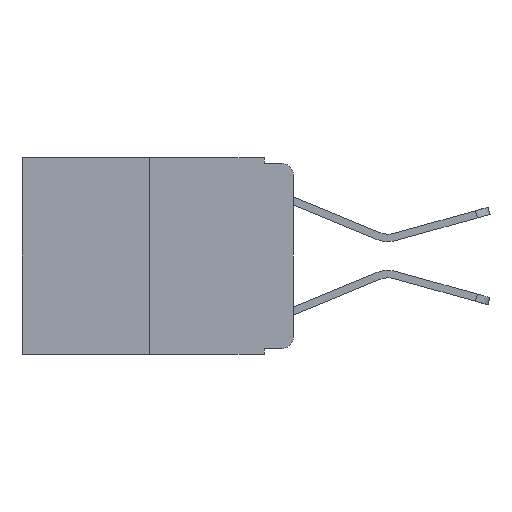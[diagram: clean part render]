
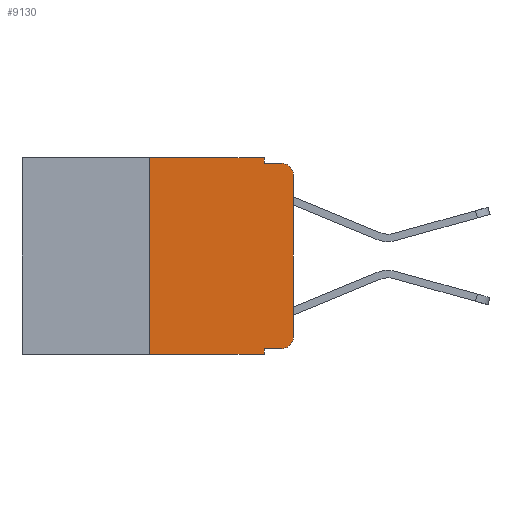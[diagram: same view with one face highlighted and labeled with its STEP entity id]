
A CAD part, left-side view. The second image highlights one B-rep face of the part: STEP entity #9130.
In plain terms, the highlighted planar face has unit normal (-1, 0, 0).
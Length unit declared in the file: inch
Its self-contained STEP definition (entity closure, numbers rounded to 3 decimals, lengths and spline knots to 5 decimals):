
#79 = EDGE_CURVE ( 'NONE', #3912, #1790, #16710, .T. ) ;
#196 = EDGE_CURVE ( 'NONE', #3220, #19184, #2141, .T. ) ;
#398 = CIRCLE ( 'NONE', #16235, 0.02 ) ;
#466 = CARTESIAN_POINT ( 'NONE',  ( 0., 0.051, -0.343 ) ) ;
#567 = LINE ( 'NONE', #5723, #11896 ) ;
#757 = CARTESIAN_POINT ( 'NONE',  ( 0., 0.02, -0.01 ) ) ;
#910 = VECTOR ( 'NONE', #4980, 39.37008 ) ;
#1705 = EDGE_CURVE ( 'NONE', #19184, #5150, #398, .T. ) ;
#1753 = CARTESIAN_POINT ( 'NONE',  ( 0., 0.02, -0.313 ) ) ;
#1790 = VERTEX_POINT ( 'NONE', #10954 ) ;
#2141 = LINE ( 'NONE', #2347, #18824 ) ;
#2221 = CIRCLE ( 'NONE', #15056, 0.02 ) ;
#2347 = CARTESIAN_POINT ( 'NONE',  ( 0., 0., 0. ) ) ;
#2667 = VERTEX_POINT ( 'NONE', #8052 ) ;
#2764 = VERTEX_POINT ( 'NONE', #10060 ) ;
#2917 = EDGE_CURVE ( 'NONE', #1790, #2667, #15469, .T. ) ;
#3115 = EDGE_CURVE ( 'NONE', #19830, #5150, #12165, .T. ) ;
#3220 = VERTEX_POINT ( 'NONE', #14313 ) ;
#3328 = DIRECTION ( 'NONE',  ( 0., 0., -1. ) ) ;
#3658 = CARTESIAN_POINT ( 'NONE',  ( 0., 0.051, -0.01 ) ) ;
#3828 = LINE ( 'NONE', #4801, #15465 ) ;
#3912 = VERTEX_POINT ( 'NONE', #14672 ) ;
#3943 = EDGE_LOOP ( 'NONE', ( #16195, #19051, #5793, #12200, #5073, #11214, #19737, #18551, #5307, #17861 ) ) ;
#4109 = VECTOR ( 'NONE', #18188, 39.37008 ) ;
#4532 = DIRECTION ( 'NONE',  ( 0., 0., -1. ) ) ;
#4801 = CARTESIAN_POINT ( 'NONE',  ( 0., 0.473, -0.343 ) ) ;
#4980 = DIRECTION ( 'NONE',  ( 0., -1., 0. ) ) ;
#5073 = ORIENTED_EDGE ( 'NONE', *, *, #2917, .F. ) ;
#5096 = LINE ( 'NONE', #11083, #910 ) ;
#5150 = VERTEX_POINT ( 'NONE', #757 ) ;
#5304 = DIRECTION ( 'NONE',  ( -1., 0., 0. ) ) ;
#5307 = ORIENTED_EDGE ( 'NONE', *, *, #13501, .T. ) ;
#5723 = CARTESIAN_POINT ( 'NONE',  ( 0., 0.051, 0. ) ) ;
#5793 = ORIENTED_EDGE ( 'NONE', *, *, #3115, .F. ) ;
#5975 = FACE_OUTER_BOUND ( 'NONE', #3943, .T. ) ;
#7239 = DIRECTION ( 'NONE',  ( 0., 0., -1. ) ) ;
#7643 = CARTESIAN_POINT ( 'NONE',  ( 0., 0., -0.03 ) ) ;
#7645 = VECTOR ( 'NONE', #17916, 39.37008 ) ;
#8049 = CARTESIAN_POINT ( 'NONE',  ( 0., 0.02, -0.03 ) ) ;
#8052 = CARTESIAN_POINT ( 'NONE',  ( 0., 0.051, 0. ) ) ;
#9011 = CARTESIAN_POINT ( 'NONE',  ( 0., 0.473, 0. ) ) ;
#9125 = CARTESIAN_POINT ( 'NONE',  ( 0., 0.473, 0. ) ) ;
#9130 = ADVANCED_FACE ( 'NONE', ( #5975 ), #10528, .F. ) ;
#9292 = EDGE_CURVE ( 'NONE', #2764, #12042, #19494, .T. ) ;
#9357 = DIRECTION ( 'NONE',  ( 0., 0., 1. ) ) ;
#10060 = CARTESIAN_POINT ( 'NONE',  ( 0., 0.051, -0.333 ) ) ;
#10528 = PLANE ( 'NONE',  #18271 ) ;
#10664 = DIRECTION ( 'NONE',  ( 0., 0., -1. ) ) ;
#10954 = CARTESIAN_POINT ( 'NONE',  ( 0., 0.25, 0. ) ) ;
#11083 = CARTESIAN_POINT ( 'NONE',  ( 0., 0.051, -0.333 ) ) ;
#11214 = ORIENTED_EDGE ( 'NONE', *, *, #79, .F. ) ;
#11450 = VECTOR ( 'NONE', #15600, 39.37008 ) ;
#11454 = VECTOR ( 'NONE', #15823, 39.37008 ) ;
#11896 = VECTOR ( 'NONE', #7239, 39.37008 ) ;
#12042 = VERTEX_POINT ( 'NONE', #466 ) ;
#12165 = LINE ( 'NONE', #18536, #7645 ) ;
#12200 = ORIENTED_EDGE ( 'NONE', *, *, #19418, .F. ) ;
#12483 = DIRECTION ( 'NONE',  ( -1., 0., 0. ) ) ;
#13286 = VERTEX_POINT ( 'NONE', #15776 ) ;
#13501 = EDGE_CURVE ( 'NONE', #2764, #13286, #5096, .T. ) ;
#13894 = DIRECTION ( 'NONE',  ( 0., -1., 0. ) ) ;
#14089 = CARTESIAN_POINT ( 'NONE',  ( 0., 0.051, 0. ) ) ;
#14313 = CARTESIAN_POINT ( 'NONE',  ( 0., 0., -0.313 ) ) ;
#14672 = CARTESIAN_POINT ( 'NONE',  ( 0., 0.25, -0.343 ) ) ;
#15056 = AXIS2_PLACEMENT_3D ( 'NONE', #1753, #12483, #3328 ) ;
#15152 = EDGE_CURVE ( 'NONE', #13286, #3220, #2221, .T. ) ;
#15465 = VECTOR ( 'NONE', #13894, 39.37008 ) ;
#15469 = LINE ( 'NONE', #9011, #11454 ) ;
#15600 = DIRECTION ( 'NONE',  ( 0., 0., -1. ) ) ;
#15776 = CARTESIAN_POINT ( 'NONE',  ( 0., 0.02, -0.333 ) ) ;
#15823 = DIRECTION ( 'NONE',  ( 0., -1., 0. ) ) ;
#16195 = ORIENTED_EDGE ( 'NONE', *, *, #196, .T. ) ;
#16235 = AXIS2_PLACEMENT_3D ( 'NONE', #8049, #5304, #4532 ) ;
#16710 = LINE ( 'NONE', #18374, #4109 ) ;
#17861 = ORIENTED_EDGE ( 'NONE', *, *, #15152, .T. ) ;
#17916 = DIRECTION ( 'NONE',  ( 0., -1., 0. ) ) ;
#18188 = DIRECTION ( 'NONE',  ( 0., 0., 1. ) ) ;
#18271 = AXIS2_PLACEMENT_3D ( 'NONE', #9125, #19716, #10664 ) ;
#18374 = CARTESIAN_POINT ( 'NONE',  ( 0., 0.25, 0. ) ) ;
#18536 = CARTESIAN_POINT ( 'NONE',  ( 0., 0.051, -0.01 ) ) ;
#18551 = ORIENTED_EDGE ( 'NONE', *, *, #9292, .F. ) ;
#18566 = EDGE_CURVE ( 'NONE', #3912, #12042, #3828, .T. ) ;
#18824 = VECTOR ( 'NONE', #9357, 39.37008 ) ;
#19051 = ORIENTED_EDGE ( 'NONE', *, *, #1705, .T. ) ;
#19184 = VERTEX_POINT ( 'NONE', #7643 ) ;
#19418 = EDGE_CURVE ( 'NONE', #2667, #19830, #567, .T. ) ;
#19494 = LINE ( 'NONE', #14089, #11450 ) ;
#19716 = DIRECTION ( 'NONE',  ( 1., 0., 0. ) ) ;
#19737 = ORIENTED_EDGE ( 'NONE', *, *, #18566, .T. ) ;
#19830 = VERTEX_POINT ( 'NONE', #3658 ) ;
